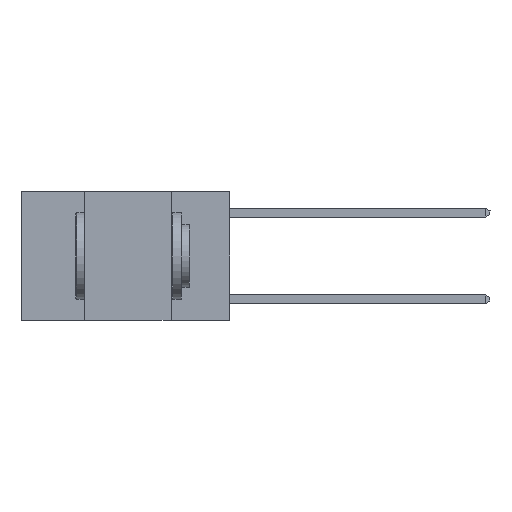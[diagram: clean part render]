
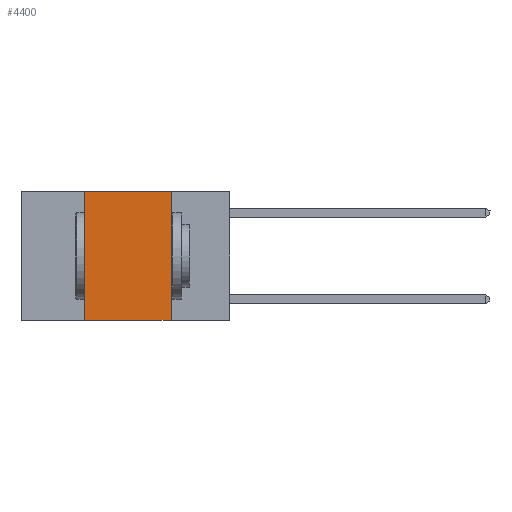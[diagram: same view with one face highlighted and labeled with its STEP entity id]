
A CAD part, left-side view. The second image highlights one B-rep face of the part: STEP entity #4400.
In plain terms, the highlighted planar face has unit normal (-1, 0, 0).
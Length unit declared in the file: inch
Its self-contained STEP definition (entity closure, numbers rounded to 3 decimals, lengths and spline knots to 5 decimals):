
#34 = ORIENTED_EDGE ( 'NONE', *, *, #24115, .F. ) ;
#342 = ORIENTED_EDGE ( 'NONE', *, *, #11528, .F. ) ;
#2650 = CARTESIAN_POINT ( 'NONE',  ( 0., 0.6, 0. ) ) ;
#4210 = LINE ( 'NONE', #23219, #9627 ) ;
#4400 = ADVANCED_FACE ( 'NONE', ( #11853 ), #7179, .F. ) ;
#4948 = DIRECTION ( 'NONE',  ( 0., 0., -1. ) ) ;
#5017 = ORIENTED_EDGE ( 'NONE', *, *, #5329, .F. ) ;
#5329 = EDGE_CURVE ( 'NONE', #26564, #14268, #24015, .T. ) ;
#5369 = ORIENTED_EDGE ( 'NONE', *, *, #6996, .T. ) ;
#5572 = CARTESIAN_POINT ( 'NONE',  ( 0., 0.17, 0. ) ) ;
#6225 = DIRECTION ( 'NONE',  ( 0., 0., 1. ) ) ;
#6996 = EDGE_CURVE ( 'NONE', #26564, #25546, #4210, .T. ) ;
#7105 = DIRECTION ( 'NONE',  ( 0., -1., 0. ) ) ;
#7179 = PLANE ( 'NONE',  #27080 ) ;
#9627 = VECTOR ( 'NONE', #7105, 39.37008 ) ;
#11528 = EDGE_CURVE ( 'NONE', #27441, #25546, #24303, .T. ) ;
#11853 = FACE_OUTER_BOUND ( 'NONE', #29098, .T. ) ;
#13141 = VECTOR ( 'NONE', #22267, 39.37008 ) ;
#14268 = VERTEX_POINT ( 'NONE', #29314 ) ;
#14877 = CARTESIAN_POINT ( 'NONE',  ( 0., 0.17, 0. ) ) ;
#17678 = CARTESIAN_POINT ( 'NONE',  ( 0., 0.17, -0.37 ) ) ;
#17927 = VECTOR ( 'NONE', #6225, 39.37008 ) ;
#18216 = VECTOR ( 'NONE', #21706, 39.37008 ) ;
#18792 = DIRECTION ( 'NONE',  ( 1., 0., 0. ) ) ;
#19960 = CARTESIAN_POINT ( 'NONE',  ( 0., 0.6, 0. ) ) ;
#19976 = LINE ( 'NONE', #19960, #13141 ) ;
#21706 = DIRECTION ( 'NONE',  ( 0., 0., -1. ) ) ;
#22267 = DIRECTION ( 'NONE',  ( 0., -1., 0. ) ) ;
#23219 = CARTESIAN_POINT ( 'NONE',  ( 0., 0.6, -0.37 ) ) ;
#23651 = CARTESIAN_POINT ( 'NONE',  ( 0., 0.42, -0.37 ) ) ;
#24015 = LINE ( 'NONE', #26878, #17927 ) ;
#24115 = EDGE_CURVE ( 'NONE', #14268, #27441, #19976, .T. ) ;
#24303 = LINE ( 'NONE', #5572, #18216 ) ;
#25546 = VERTEX_POINT ( 'NONE', #17678 ) ;
#26564 = VERTEX_POINT ( 'NONE', #23651 ) ;
#26878 = CARTESIAN_POINT ( 'NONE',  ( 0., 0.42, 0. ) ) ;
#27080 = AXIS2_PLACEMENT_3D ( 'NONE', #2650, #18792, #4948 ) ;
#27441 = VERTEX_POINT ( 'NONE', #14877 ) ;
#29098 = EDGE_LOOP ( 'NONE', ( #342, #34, #5017, #5369 ) ) ;
#29314 = CARTESIAN_POINT ( 'NONE',  ( 0., 0.42, 0. ) ) ;
